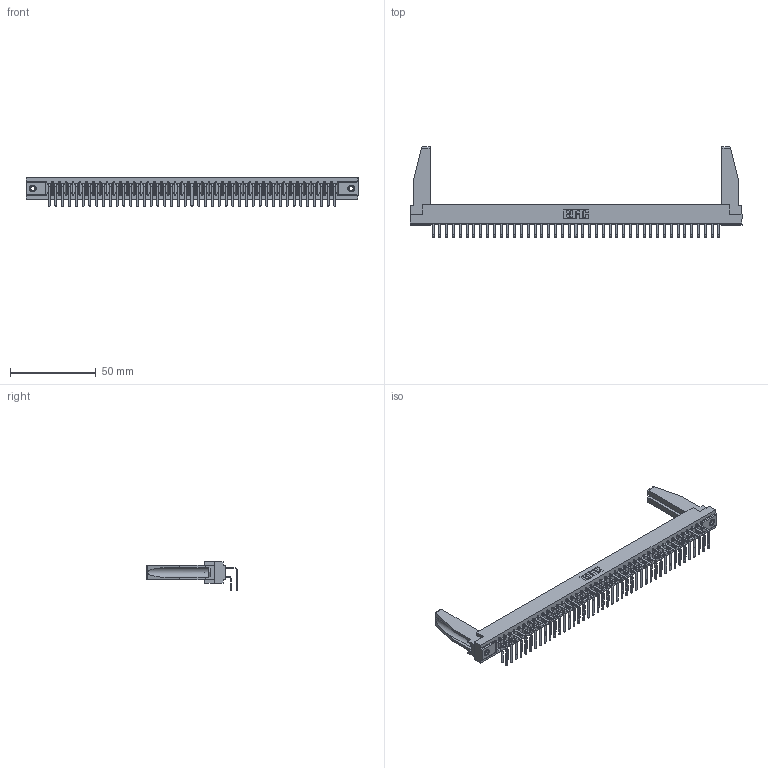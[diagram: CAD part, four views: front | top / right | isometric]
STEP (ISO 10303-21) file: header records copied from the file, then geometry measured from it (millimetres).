
FILE_DESCRIPTION (( 'STEP AP203' ), '1' );
FILE_NAME ('357-086-558-278.STEP', '2019-09-19T19:37:20', ( '' ), ( '' ), 'SwSTEP 2.0', 'SolidWorks 2016', '' );
FILE_SCHEMA (( 'CONFIG_CONTROL_DESIGN' ));
Length unit declared in the file: inch
Products named in the file (6): 357-086-558-278; 345-250-001_345-250-001-102; 307-220-078; 307 Part_.156 Dia Mounting Holes; 307-290-001_558 559 - 1 (Single); 307-290-001_558 - 2 (Single)
Assembly tree (91 placements, depth 2):
  357-086-558-278
    307 Part_.156 Dia Mounting Holes
    307-290-001_558 559 - 1 (Single)  x43
    307-290-001_558 - 2 (Single)  x43
    307-220-078  x2
    345-250-001_345-250-001-102  x2
Bounding box: 193.4 x 52.67 x 16.8 mm (x, y, z)
Volume: 24947 mm3; surface area: 31705.8 mm2
Topology: 91 solids, 91 shells, 4592 faces, 12865 edges, 8334 vertices
Faces by surface type: plane 2992, cylinder 1496, sphere 88, cone 12, torus 4
Entity records: 42002 total; most frequent: CARTESIAN_POINT 6883, ORIENTED_EDGE 6780, DIRECTION 6694, EDGE_CURVE 3390, LINE 2604, VECTOR 2604, VERTEX_POINT 2192, AXIS2_PLACEMENT_3D 2045
